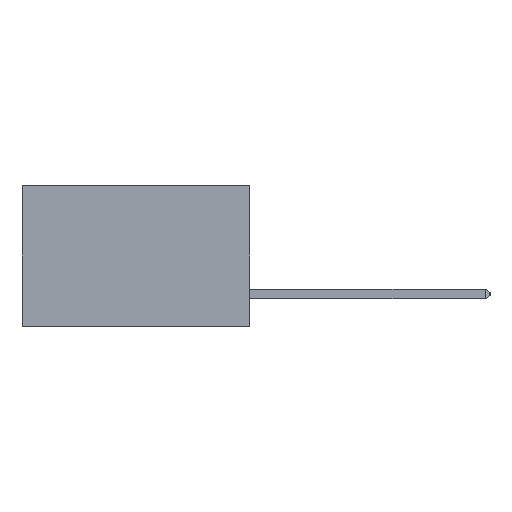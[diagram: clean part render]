
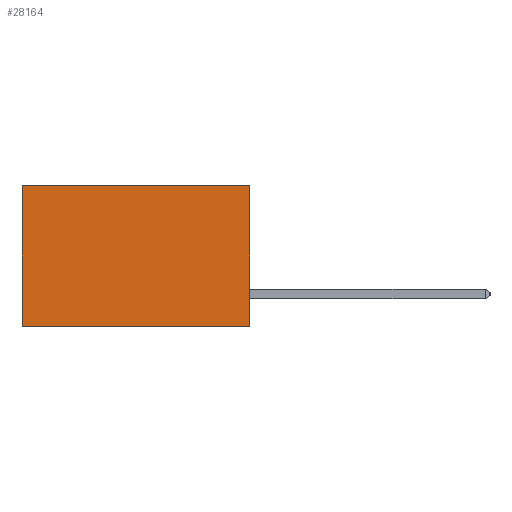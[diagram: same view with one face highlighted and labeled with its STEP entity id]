
A CAD part, left-side view. The second image highlights one B-rep face of the part: STEP entity #28164.
In plain terms, the highlighted planar face has unit normal (-1, 0, 0).
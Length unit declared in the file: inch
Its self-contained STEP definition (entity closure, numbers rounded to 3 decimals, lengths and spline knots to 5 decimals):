
#89 = CARTESIAN_POINT ( 'NONE',  ( 0.2875, 0., -0.37 ) ) ;
#980 = EDGE_LOOP ( 'NONE', ( #32521, #25901, #8800, #2490 ) ) ;
#1914 = CARTESIAN_POINT ( 'NONE',  ( 0.2875, 0., -0.37 ) ) ;
#2490 = ORIENTED_EDGE ( 'NONE', *, *, #25207, .T. ) ;
#3003 = DIRECTION ( 'NONE',  ( 0., 1., 0. ) ) ;
#5971 = DIRECTION ( 'NONE',  ( 0., 1., 0. ) ) ;
#6604 = VECTOR ( 'NONE', #26132, 39.37008 ) ;
#7376 = VERTEX_POINT ( 'NONE', #8660 ) ;
#8660 = CARTESIAN_POINT ( 'NONE',  ( 0.2875, 0., 0. ) ) ;
#8800 = ORIENTED_EDGE ( 'NONE', *, *, #35405, .F. ) ;
#10223 = DIRECTION ( 'NONE',  ( 0., 0., -1. ) ) ;
#10994 = VECTOR ( 'NONE', #3003, 39.37008 ) ;
#11771 = CARTESIAN_POINT ( 'NONE',  ( 0.2875, 0., 0. ) ) ;
#12567 = VERTEX_POINT ( 'NONE', #1914 ) ;
#14614 = DIRECTION ( 'NONE',  ( 0., 0., -1. ) ) ;
#14803 = CARTESIAN_POINT ( 'NONE',  ( 0.2875, 0.6, 0. ) ) ;
#15145 = LINE ( 'NONE', #14803, #6604 ) ;
#17054 = CARTESIAN_POINT ( 'NONE',  ( 0.2875, 0.6, -0.37 ) ) ;
#17325 = VERTEX_POINT ( 'NONE', #17054 ) ;
#17364 = PLANE ( 'NONE',  #24332 ) ;
#18165 = VECTOR ( 'NONE', #5971, 39.37008 ) ;
#19461 = LINE ( 'NONE', #89, #10994 ) ;
#20263 = CARTESIAN_POINT ( 'NONE',  ( 0.2875, 0., 0. ) ) ;
#23735 = LINE ( 'NONE', #35693, #30315 ) ;
#24332 = AXIS2_PLACEMENT_3D ( 'NONE', #11771, #31504, #14614 ) ;
#25207 = EDGE_CURVE ( 'NONE', #7376, #27028, #26624, .T. ) ;
#25850 = EDGE_CURVE ( 'NONE', #12567, #17325, #19461, .T. ) ;
#25901 = ORIENTED_EDGE ( 'NONE', *, *, #25850, .F. ) ;
#26132 = DIRECTION ( 'NONE',  ( 0., 0., -1. ) ) ;
#26624 = LINE ( 'NONE', #20263, #18165 ) ;
#27028 = VERTEX_POINT ( 'NONE', #35060 ) ;
#28164 = ADVANCED_FACE ( 'NONE', ( #28675 ), #17364, .F. ) ;
#28675 = FACE_OUTER_BOUND ( 'NONE', #980, .T. ) ;
#30315 = VECTOR ( 'NONE', #10223, 39.37008 ) ;
#31072 = EDGE_CURVE ( 'NONE', #27028, #17325, #15145, .T. ) ;
#31504 = DIRECTION ( 'NONE',  ( 1., 0., 0. ) ) ;
#32521 = ORIENTED_EDGE ( 'NONE', *, *, #31072, .T. ) ;
#35060 = CARTESIAN_POINT ( 'NONE',  ( 0.2875, 0.6, 0. ) ) ;
#35405 = EDGE_CURVE ( 'NONE', #7376, #12567, #23735, .T. ) ;
#35693 = CARTESIAN_POINT ( 'NONE',  ( 0.2875, 0., 0. ) ) ;
